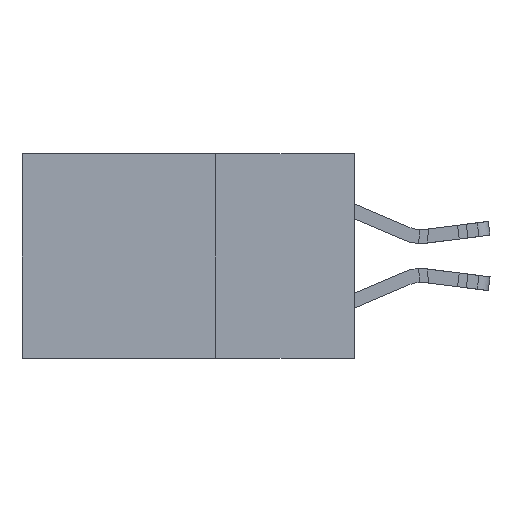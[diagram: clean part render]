
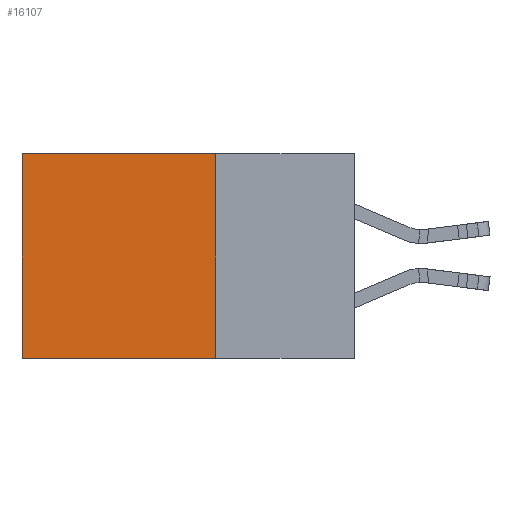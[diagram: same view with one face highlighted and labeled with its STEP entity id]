
A CAD part, left-side view. The second image highlights one B-rep face of the part: STEP entity #16107.
In plain terms, the highlighted planar face has unit normal (-1, 0, 0).
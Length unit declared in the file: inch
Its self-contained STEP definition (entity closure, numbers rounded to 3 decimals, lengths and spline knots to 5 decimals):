
#668 = VERTEX_POINT ( 'NONE', #4788 ) ;
#3130 = EDGE_CURVE ( 'NONE', #24779, #9435, #4043, .T. ) ;
#4043 = LINE ( 'NONE', #23387, #20972 ) ;
#4258 = CARTESIAN_POINT ( 'NONE',  ( 0.2615, 0.6, -0.37 ) ) ;
#4788 = CARTESIAN_POINT ( 'NONE',  ( 0.2615, 0.25, 0. ) ) ;
#5319 = EDGE_CURVE ( 'NONE', #668, #23470, #26311, .T. ) ;
#7592 = ORIENTED_EDGE ( 'NONE', *, *, #5319, .T. ) ;
#7896 = CARTESIAN_POINT ( 'NONE',  ( 0.2615, 0.6, 0. ) ) ;
#7966 = PLANE ( 'NONE',  #25248 ) ;
#9435 = VERTEX_POINT ( 'NONE', #20843 ) ;
#9559 = VECTOR ( 'NONE', #10153, 39.37008 ) ;
#9873 = EDGE_CURVE ( 'NONE', #668, #24779, #12388, .T. ) ;
#10147 = CARTESIAN_POINT ( 'NONE',  ( 0.2615, 0.25, 0. ) ) ;
#10153 = DIRECTION ( 'NONE',  ( 0., 1., 0. ) ) ;
#10156 = DIRECTION ( 'NONE',  ( 0., 0., -1. ) ) ;
#10968 = VECTOR ( 'NONE', #19130, 39.37008 ) ;
#11650 = LINE ( 'NONE', #4258, #10968 ) ;
#12388 = LINE ( 'NONE', #14175, #22845 ) ;
#12691 = ORIENTED_EDGE ( 'NONE', *, *, #24523, .T. ) ;
#12817 = ORIENTED_EDGE ( 'NONE', *, *, #3130, .F. ) ;
#14175 = CARTESIAN_POINT ( 'NONE',  ( 0.2615, 0.25, -0.37 ) ) ;
#15754 = CARTESIAN_POINT ( 'NONE',  ( 0.2615, 0.25, -0.37 ) ) ;
#16107 = ADVANCED_FACE ( 'NONE', ( #18035 ), #7966, .F. ) ;
#16530 = EDGE_LOOP ( 'NONE', ( #12691, #12817, #17631, #7592 ) ) ;
#17631 = ORIENTED_EDGE ( 'NONE', *, *, #9873, .F. ) ;
#18035 = FACE_OUTER_BOUND ( 'NONE', #16530, .T. ) ;
#18339 = DIRECTION ( 'NONE',  ( 0., 0., -1. ) ) ;
#19130 = DIRECTION ( 'NONE',  ( 0., 0., -1. ) ) ;
#20843 = CARTESIAN_POINT ( 'NONE',  ( 0.2615, 0.6, -0.37 ) ) ;
#20972 = VECTOR ( 'NONE', #23229, 39.37008 ) ;
#22758 = DIRECTION ( 'NONE',  ( 1., 0., 0. ) ) ;
#22845 = VECTOR ( 'NONE', #18339, 39.37008 ) ;
#23229 = DIRECTION ( 'NONE',  ( 0., 1., 0. ) ) ;
#23387 = CARTESIAN_POINT ( 'NONE',  ( 0.2615, 0.25, -0.37 ) ) ;
#23470 = VERTEX_POINT ( 'NONE', #7896 ) ;
#24523 = EDGE_CURVE ( 'NONE', #23470, #9435, #11650, .T. ) ;
#24759 = CARTESIAN_POINT ( 'NONE',  ( 0.2615, 0.25, -0.37 ) ) ;
#24779 = VERTEX_POINT ( 'NONE', #15754 ) ;
#25248 = AXIS2_PLACEMENT_3D ( 'NONE', #24759, #22758, #10156 ) ;
#26311 = LINE ( 'NONE', #10147, #9559 ) ;
